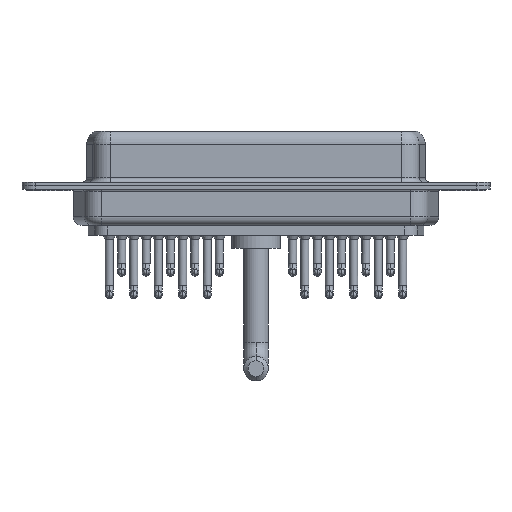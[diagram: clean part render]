
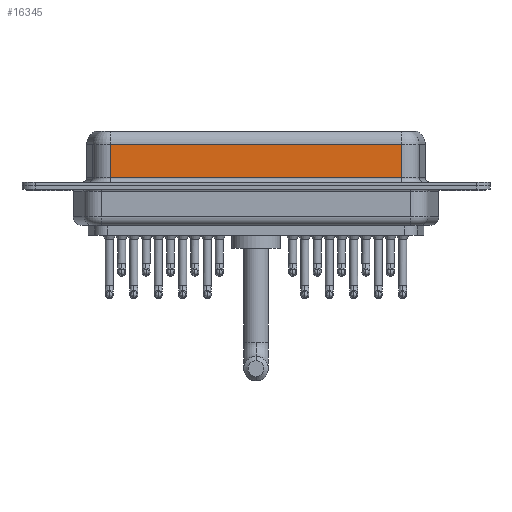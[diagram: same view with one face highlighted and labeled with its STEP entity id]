
A CAD part, front view. The second image highlights one B-rep face of the part: STEP entity #16345.
In plain terms, the highlighted planar face has unit normal (0, -1, 0).
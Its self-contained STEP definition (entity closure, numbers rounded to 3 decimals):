
#903 = FACE_OUTER_BOUND ( 'NONE', #14463, .T. ) ;
#1757 = LINE ( 'NONE', #2171, #10894 ) ;
#2171 = CARTESIAN_POINT ( 'NONE',  ( 40.037, -3.95, 6.4 ) ) ;
#4391 = EDGE_CURVE ( 'NONE', #4403, #18966, #8201, .T. ) ;
#4403 = VERTEX_POINT ( 'NONE', #16302 ) ;
#4848 = VERTEX_POINT ( 'NONE', #11032 ) ;
#5431 = DIRECTION ( 'NONE',  ( 0., 0., -1. ) ) ;
#7129 = DIRECTION ( 'NONE',  ( 0., 1., 0. ) ) ;
#7262 = VECTOR ( 'NONE', #5431, 1000. ) ;
#8201 = LINE ( 'NONE', #17877, #13709 ) ;
#8304 = DIRECTION ( 'NONE',  ( -1., 0., 0. ) ) ;
#8841 = EDGE_CURVE ( 'NONE', #10702, #18966, #1757, .T. ) ;
#10302 = EDGE_CURVE ( 'NONE', #10702, #4848, #11353, .T. ) ;
#10458 = EDGE_CURVE ( 'NONE', #4848, #4403, #11767, .T. ) ;
#10702 = VERTEX_POINT ( 'NONE', #12501 ) ;
#10894 = VECTOR ( 'NONE', #18181, 1000. ) ;
#11032 = CARTESIAN_POINT ( 'NONE',  ( 7.013, -3.95, 4.65 ) ) ;
#11353 = LINE ( 'NONE', #13247, #14989 ) ;
#11742 = ORIENTED_EDGE ( 'NONE', *, *, #4391, .T. ) ;
#11767 = LINE ( 'NONE', #18276, #7262 ) ;
#12188 = PLANE ( 'NONE',  #13105 ) ;
#12501 = CARTESIAN_POINT ( 'NONE',  ( 40.037, -3.95, 4.65 ) ) ;
#12841 = DIRECTION ( 'NONE',  ( 1., 0., 0. ) ) ;
#13105 = AXIS2_PLACEMENT_3D ( 'NONE', #16919, #7129, #15229 ) ;
#13247 = CARTESIAN_POINT ( 'NONE',  ( 40.037, -3.95, 4.65 ) ) ;
#13527 = ORIENTED_EDGE ( 'NONE', *, *, #10302, .T. ) ;
#13709 = VECTOR ( 'NONE', #12841, 1000. ) ;
#14463 = EDGE_LOOP ( 'NONE', ( #18319, #13527, #20219, #11742 ) ) ;
#14989 = VECTOR ( 'NONE', #8304, 1000. ) ;
#15229 = DIRECTION ( 'NONE',  ( 0., 0., 1. ) ) ;
#16302 = CARTESIAN_POINT ( 'NONE',  ( 7.013, -3.95, 0.9 ) ) ;
#16345 = ADVANCED_FACE ( 'NONE', ( #903 ), #12188, .F. ) ;
#16919 = CARTESIAN_POINT ( 'NONE',  ( 40.037, -3.95, 6.4 ) ) ;
#17402 = CARTESIAN_POINT ( 'NONE',  ( 40.037, -3.95, 0.9 ) ) ;
#17877 = CARTESIAN_POINT ( 'NONE',  ( 40.037, -3.95, 0.9 ) ) ;
#18181 = DIRECTION ( 'NONE',  ( 0., 0., -1. ) ) ;
#18276 = CARTESIAN_POINT ( 'NONE',  ( 7.013, -3.95, 6.4 ) ) ;
#18319 = ORIENTED_EDGE ( 'NONE', *, *, #8841, .F. ) ;
#18966 = VERTEX_POINT ( 'NONE', #17402 ) ;
#20219 = ORIENTED_EDGE ( 'NONE', *, *, #10458, .T. ) ;
